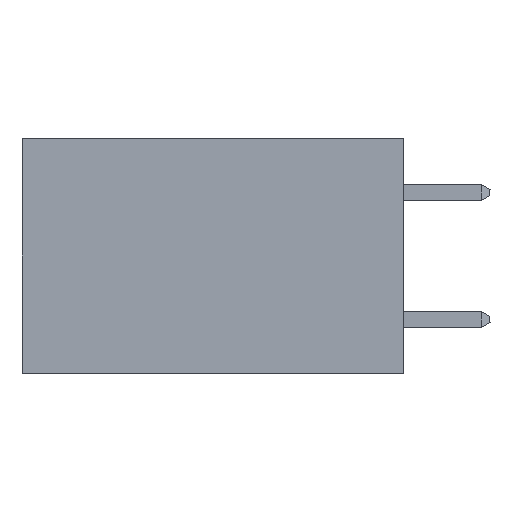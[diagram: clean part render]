
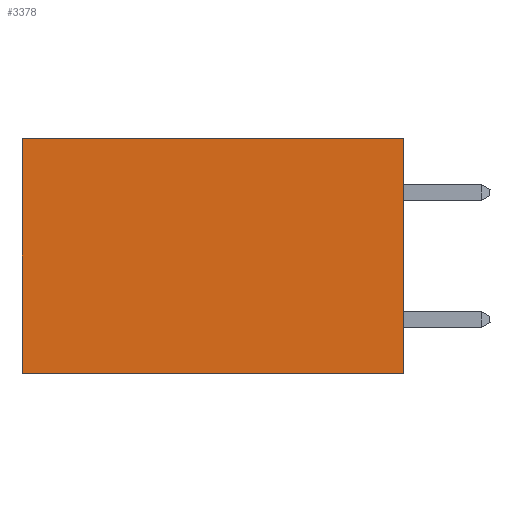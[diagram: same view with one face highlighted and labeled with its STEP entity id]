
A CAD part, left-side view. The second image highlights one B-rep face of the part: STEP entity #3378.
In plain terms, the highlighted planar face has unit normal (-1, 0, 0).
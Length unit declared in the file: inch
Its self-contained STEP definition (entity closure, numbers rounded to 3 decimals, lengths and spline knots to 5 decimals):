
#2339 = DIRECTION ( 'NONE',  ( 0., 0., -1. ) ) ;
#3378 = ADVANCED_FACE ( 'NONE', ( #7259 ), #18852, .F. ) ;
#3492 = CARTESIAN_POINT ( 'NONE',  ( 0.2875, 0., 0. ) ) ;
#5635 = LINE ( 'NONE', #7850, #36893 ) ;
#6472 = VECTOR ( 'NONE', #23324, 39.37008 ) ;
#7259 = FACE_OUTER_BOUND ( 'NONE', #31592, .T. ) ;
#7850 = CARTESIAN_POINT ( 'NONE',  ( 0.2875, 0., 0. ) ) ;
#10277 = ORIENTED_EDGE ( 'NONE', *, *, #35234, .F. ) ;
#10665 = VERTEX_POINT ( 'NONE', #12376 ) ;
#12068 = AXIS2_PLACEMENT_3D ( 'NONE', #3492, #29164, #2339 ) ;
#12376 = CARTESIAN_POINT ( 'NONE',  ( 0.2875, 0., 0. ) ) ;
#12967 = DIRECTION ( 'NONE',  ( 0., 1., 0. ) ) ;
#13521 = CARTESIAN_POINT ( 'NONE',  ( 0.2875, 0.6, 0. ) ) ;
#14024 = LINE ( 'NONE', #13521, #37108 ) ;
#15553 = ORIENTED_EDGE ( 'NONE', *, *, #30569, .T. ) ;
#16653 = DIRECTION ( 'NONE',  ( 0., 0., -1. ) ) ;
#17175 = CARTESIAN_POINT ( 'NONE',  ( 0.2875, 0., 0. ) ) ;
#18852 = PLANE ( 'NONE',  #12068 ) ;
#19623 = VERTEX_POINT ( 'NONE', #31617 ) ;
#20235 = DIRECTION ( 'NONE',  ( 0., 0., -1. ) ) ;
#21105 = LINE ( 'NONE', #27992, #36033 ) ;
#21544 = EDGE_CURVE ( 'NONE', #34717, #19623, #14024, .T. ) ;
#21730 = ORIENTED_EDGE ( 'NONE', *, *, #28436, .F. ) ;
#23181 = CARTESIAN_POINT ( 'NONE',  ( 0.2875, 0.6, 0. ) ) ;
#23324 = DIRECTION ( 'NONE',  ( 0., 1., 0. ) ) ;
#26022 = ORIENTED_EDGE ( 'NONE', *, *, #21544, .T. ) ;
#27739 = VERTEX_POINT ( 'NONE', #28040 ) ;
#27992 = CARTESIAN_POINT ( 'NONE',  ( 0.2875, 0., -0.37 ) ) ;
#28040 = CARTESIAN_POINT ( 'NONE',  ( 0.2875, 0., -0.37 ) ) ;
#28436 = EDGE_CURVE ( 'NONE', #27739, #19623, #21105, .T. ) ;
#29164 = DIRECTION ( 'NONE',  ( 1., 0., 0. ) ) ;
#30569 = EDGE_CURVE ( 'NONE', #10665, #34717, #30731, .T. ) ;
#30731 = LINE ( 'NONE', #17175, #6472 ) ;
#31592 = EDGE_LOOP ( 'NONE', ( #26022, #21730, #10277, #15553 ) ) ;
#31617 = CARTESIAN_POINT ( 'NONE',  ( 0.2875, 0.6, -0.37 ) ) ;
#34717 = VERTEX_POINT ( 'NONE', #23181 ) ;
#35234 = EDGE_CURVE ( 'NONE', #10665, #27739, #5635, .T. ) ;
#36033 = VECTOR ( 'NONE', #12967, 39.37008 ) ;
#36893 = VECTOR ( 'NONE', #20235, 39.37008 ) ;
#37108 = VECTOR ( 'NONE', #16653, 39.37008 ) ;
